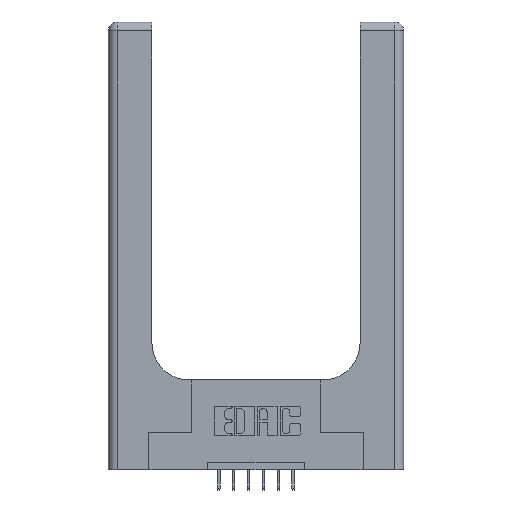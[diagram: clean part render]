
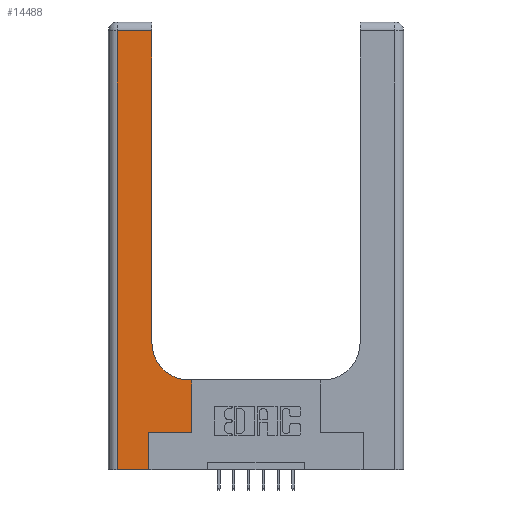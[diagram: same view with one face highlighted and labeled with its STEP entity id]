
A CAD part, top view. The second image highlights one B-rep face of the part: STEP entity #14488.
In plain terms, the highlighted planar face has unit normal (0, 0, 1).
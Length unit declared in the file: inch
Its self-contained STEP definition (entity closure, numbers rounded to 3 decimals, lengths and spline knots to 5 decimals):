
#120 = LINE ( 'NONE', #5920, #14472 ) ;
#184 = LINE ( 'NONE', #3779, #6742 ) ;
#231 = ORIENTED_EDGE ( 'NONE', *, *, #8923, .T. ) ;
#492 = EDGE_CURVE ( 'NONE', #8517, #5265, #184, .T. ) ;
#641 = CARTESIAN_POINT ( 'NONE',  ( 0.2915, 0.85, 0.37 ) ) ;
#672 = CARTESIAN_POINT ( 'NONE',  ( 0.06, 0., 0.37 ) ) ;
#882 = LINE ( 'NONE', #5433, #5192 ) ;
#1122 = DIRECTION ( 'NONE',  ( 0., 1., 0. ) ) ;
#1193 = CARTESIAN_POINT ( 'NONE',  ( 0.269, 0.25, 0.37 ) ) ;
#1657 = CARTESIAN_POINT ( 'NONE',  ( 0., 0., 0.37 ) ) ;
#2021 = EDGE_CURVE ( 'NONE', #5874, #8517, #5230, .T. ) ;
#2149 = VECTOR ( 'NONE', #8118, 39.37008 ) ;
#2254 = ORIENTED_EDGE ( 'NONE', *, *, #7762, .T. ) ;
#2653 = ORIENTED_EDGE ( 'NONE', *, *, #12694, .T. ) ;
#2836 = DIRECTION ( 'NONE',  ( 1., 0., 0. ) ) ;
#3531 = DIRECTION ( 'NONE',  ( -1., 0., 0. ) ) ;
#3544 = CARTESIAN_POINT ( 'NONE',  ( 0.269, 0., 0.37 ) ) ;
#3779 = CARTESIAN_POINT ( 'NONE',  ( 0.2915, 0.6, 0.37 ) ) ;
#3945 = CARTESIAN_POINT ( 'NONE',  ( 0.5415, 0.85, 0.37 ) ) ;
#4121 = DIRECTION ( 'NONE',  ( 0., 1., 0. ) ) ;
#4197 = ORIENTED_EDGE ( 'NONE', *, *, #2021, .T. ) ;
#4449 = ORIENTED_EDGE ( 'NONE', *, *, #10211, .T. ) ;
#4668 = CIRCLE ( 'NONE', #13897, 0.25 ) ;
#5086 = CARTESIAN_POINT ( 'NONE',  ( 0.269, 0.25, 0.37 ) ) ;
#5192 = VECTOR ( 'NONE', #7819, 39.37008 ) ;
#5230 = LINE ( 'NONE', #14352, #9169 ) ;
#5265 = VERTEX_POINT ( 'NONE', #7108 ) ;
#5433 = CARTESIAN_POINT ( 'NONE',  ( 0.2915, 3., 0.37 ) ) ;
#5440 = EDGE_CURVE ( 'NONE', #5670, #10463, #7771, .T. ) ;
#5596 = PLANE ( 'NONE',  #7390 ) ;
#5670 = VERTEX_POINT ( 'NONE', #3544 ) ;
#5874 = VERTEX_POINT ( 'NONE', #9902 ) ;
#5920 = CARTESIAN_POINT ( 'NONE',  ( 0.06, 3., 0.37 ) ) ;
#6339 = EDGE_CURVE ( 'NONE', #5265, #9248, #4668, .T. ) ;
#6742 = VECTOR ( 'NONE', #8311, 39.37008 ) ;
#6799 = ORIENTED_EDGE ( 'NONE', *, *, #12313, .T. ) ;
#6980 = VERTEX_POINT ( 'NONE', #672 ) ;
#7108 = CARTESIAN_POINT ( 'NONE',  ( 0.5415, 0.6, 0.37 ) ) ;
#7283 = VECTOR ( 'NONE', #10836, 39.37008 ) ;
#7390 = AXIS2_PLACEMENT_3D ( 'NONE', #12593, #9168, #3531 ) ;
#7762 = EDGE_CURVE ( 'NONE', #6980, #5670, #11732, .T. ) ;
#7771 = LINE ( 'NONE', #10980, #11579 ) ;
#7819 = DIRECTION ( 'NONE',  ( 0., 1., 0. ) ) ;
#8118 = DIRECTION ( 'NONE',  ( -1., 0., 0. ) ) ;
#8311 = DIRECTION ( 'NONE',  ( -1., 0., 0. ) ) ;
#8517 = VERTEX_POINT ( 'NONE', #12666 ) ;
#8923 = EDGE_CURVE ( 'NONE', #9248, #13912, #882, .T. ) ;
#9168 = DIRECTION ( 'NONE',  ( 0., 0., -1. ) ) ;
#9169 = VECTOR ( 'NONE', #4121, 39.37008 ) ;
#9248 = VERTEX_POINT ( 'NONE', #641 ) ;
#9646 = CARTESIAN_POINT ( 'NONE',  ( 0.06, 2.94, 0.37 ) ) ;
#9902 = CARTESIAN_POINT ( 'NONE',  ( 0.5585, 0.25, 0.37 ) ) ;
#10211 = EDGE_CURVE ( 'NONE', #10463, #5874, #11336, .T. ) ;
#10227 = DIRECTION ( 'NONE',  ( 1., 0., 0. ) ) ;
#10295 = FACE_OUTER_BOUND ( 'NONE', #10516, .T. ) ;
#10463 = VERTEX_POINT ( 'NONE', #5086 ) ;
#10516 = EDGE_LOOP ( 'NONE', ( #231, #6799, #2653, #2254, #13971, #4449, #4197, #14464, #13757 ) ) ;
#10836 = DIRECTION ( 'NONE',  ( 1., 0., 0. ) ) ;
#10980 = CARTESIAN_POINT ( 'NONE',  ( 0.269, 0., 0.37 ) ) ;
#11271 = CARTESIAN_POINT ( 'NONE',  ( 0.2915, 2.94, 0.37 ) ) ;
#11336 = LINE ( 'NONE', #1193, #12334 ) ;
#11579 = VECTOR ( 'NONE', #1122, 39.37008 ) ;
#11665 = DIRECTION ( 'NONE',  ( 0., -1., 0. ) ) ;
#11732 = LINE ( 'NONE', #1657, #7283 ) ;
#12313 = EDGE_CURVE ( 'NONE', #13912, #13797, #14159, .T. ) ;
#12334 = VECTOR ( 'NONE', #10227, 39.37008 ) ;
#12593 = CARTESIAN_POINT ( 'NONE',  ( 0., 3., 0.37 ) ) ;
#12666 = CARTESIAN_POINT ( 'NONE',  ( 0.5585, 0.6, 0.37 ) ) ;
#12694 = EDGE_CURVE ( 'NONE', #13797, #6980, #120, .T. ) ;
#12712 = CARTESIAN_POINT ( 'NONE',  ( 0., 2.94, 0.37 ) ) ;
#13009 = DIRECTION ( 'NONE',  ( 0., 0., -1. ) ) ;
#13757 = ORIENTED_EDGE ( 'NONE', *, *, #6339, .T. ) ;
#13797 = VERTEX_POINT ( 'NONE', #9646 ) ;
#13897 = AXIS2_PLACEMENT_3D ( 'NONE', #3945, #13009, #2836 ) ;
#13912 = VERTEX_POINT ( 'NONE', #11271 ) ;
#13971 = ORIENTED_EDGE ( 'NONE', *, *, #5440, .T. ) ;
#14159 = LINE ( 'NONE', #12712, #2149 ) ;
#14352 = CARTESIAN_POINT ( 'NONE',  ( 0.5585, 0.25, 0.37 ) ) ;
#14464 = ORIENTED_EDGE ( 'NONE', *, *, #492, .T. ) ;
#14472 = VECTOR ( 'NONE', #11665, 39.37008 ) ;
#14488 = ADVANCED_FACE ( 'NONE', ( #10295 ), #5596, .F. ) ;
